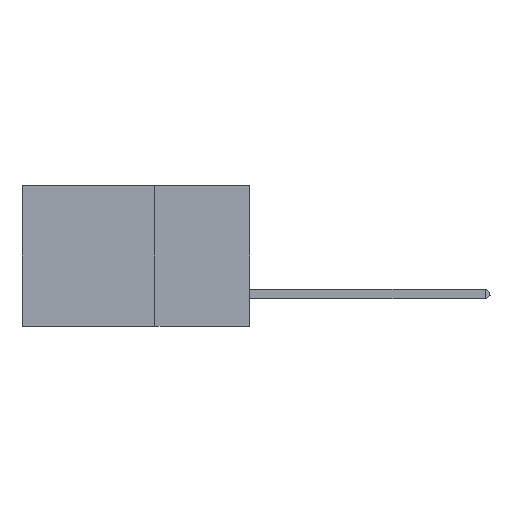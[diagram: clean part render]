
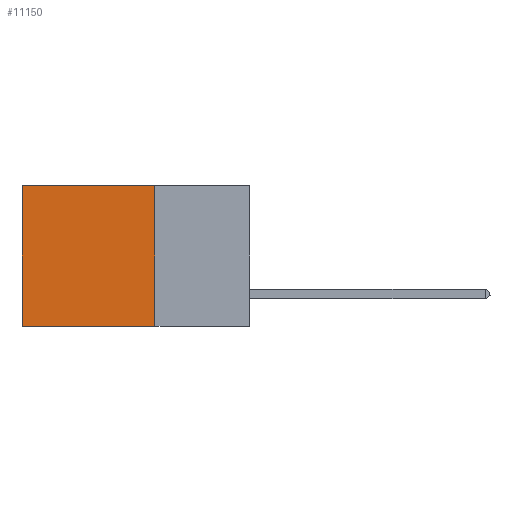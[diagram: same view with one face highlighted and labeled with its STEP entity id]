
A CAD part, left-side view. The second image highlights one B-rep face of the part: STEP entity #11150.
In plain terms, the highlighted planar face has unit normal (-1, 0, 0).
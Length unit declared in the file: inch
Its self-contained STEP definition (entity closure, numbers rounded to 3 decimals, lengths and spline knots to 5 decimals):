
#1118 = CARTESIAN_POINT ( 'NONE',  ( 0.2875, 0.25, 0. ) ) ;
#1922 = VERTEX_POINT ( 'NONE', #19628 ) ;
#2422 = LINE ( 'NONE', #14025, #5336 ) ;
#3784 = CARTESIAN_POINT ( 'NONE',  ( 0.2875, 0.6, 0. ) ) ;
#4412 = VECTOR ( 'NONE', #15482, 39.37008 ) ;
#5336 = VECTOR ( 'NONE', #15986, 39.37008 ) ;
#6387 = FACE_OUTER_BOUND ( 'NONE', #6852, .T. ) ;
#6746 = EDGE_CURVE ( 'NONE', #17310, #12430, #21842, .T. ) ;
#6852 = EDGE_LOOP ( 'NONE', ( #14667, #7324, #25215, #11698 ) ) ;
#7315 = VECTOR ( 'NONE', #23392, 39.37008 ) ;
#7324 = ORIENTED_EDGE ( 'NONE', *, *, #6746, .F. ) ;
#7654 = EDGE_CURVE ( 'NONE', #13340, #12430, #26644, .T. ) ;
#8273 = CARTESIAN_POINT ( 'NONE',  ( 0.2875, 0.6, -0.37 ) ) ;
#9636 = DIRECTION ( 'NONE',  ( 0., 0., -1. ) ) ;
#9881 = LINE ( 'NONE', #1118, #4412 ) ;
#10491 = VECTOR ( 'NONE', #26208, 39.37008 ) ;
#11150 = ADVANCED_FACE ( 'NONE', ( #6387 ), #12056, .F. ) ;
#11606 = AXIS2_PLACEMENT_3D ( 'NONE', #26492, #16188, #9636 ) ;
#11698 = ORIENTED_EDGE ( 'NONE', *, *, #16675, .T. ) ;
#12056 = PLANE ( 'NONE',  #11606 ) ;
#12430 = VERTEX_POINT ( 'NONE', #8273 ) ;
#13054 = CARTESIAN_POINT ( 'NONE',  ( 0.2875, 0.25, -0.37 ) ) ;
#13066 = CARTESIAN_POINT ( 'NONE',  ( 0.2875, 0.25, -0.37 ) ) ;
#13340 = VERTEX_POINT ( 'NONE', #22606 ) ;
#14025 = CARTESIAN_POINT ( 'NONE',  ( 0.2875, 0.25, 0. ) ) ;
#14667 = ORIENTED_EDGE ( 'NONE', *, *, #7654, .T. ) ;
#15482 = DIRECTION ( 'NONE',  ( 0., 1., 0. ) ) ;
#15986 = DIRECTION ( 'NONE',  ( 0., 0., -1. ) ) ;
#16188 = DIRECTION ( 'NONE',  ( 1., 0., 0. ) ) ;
#16675 = EDGE_CURVE ( 'NONE', #1922, #13340, #9881, .T. ) ;
#17310 = VERTEX_POINT ( 'NONE', #13054 ) ;
#17484 = EDGE_CURVE ( 'NONE', #1922, #17310, #2422, .T. ) ;
#19628 = CARTESIAN_POINT ( 'NONE',  ( 0.2875, 0.25, 0. ) ) ;
#21842 = LINE ( 'NONE', #13066, #7315 ) ;
#22606 = CARTESIAN_POINT ( 'NONE',  ( 0.2875, 0.6, 0. ) ) ;
#23392 = DIRECTION ( 'NONE',  ( 0., 1., 0. ) ) ;
#25215 = ORIENTED_EDGE ( 'NONE', *, *, #17484, .F. ) ;
#26208 = DIRECTION ( 'NONE',  ( 0., 0., -1. ) ) ;
#26492 = CARTESIAN_POINT ( 'NONE',  ( 0.2875, 0.25, 0. ) ) ;
#26644 = LINE ( 'NONE', #3784, #10491 ) ;
